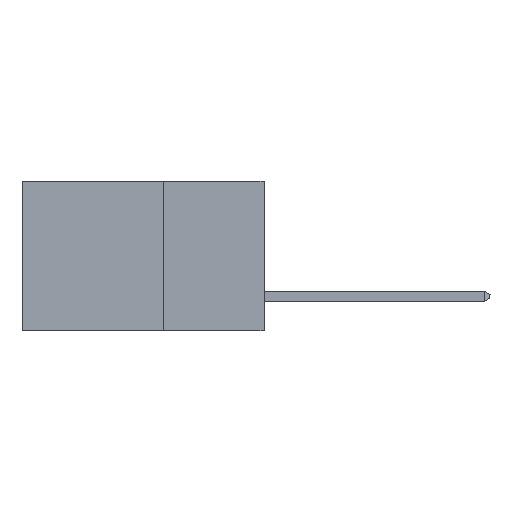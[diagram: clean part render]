
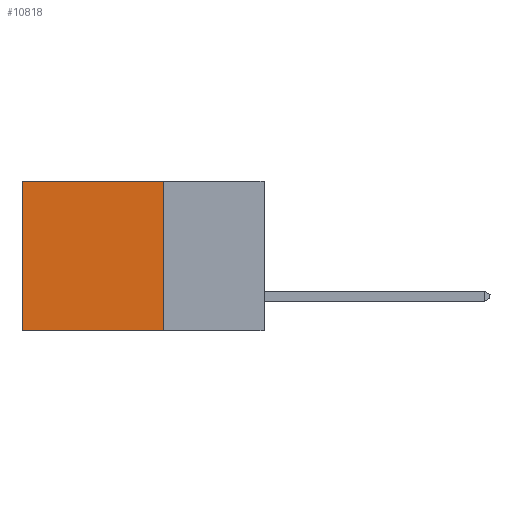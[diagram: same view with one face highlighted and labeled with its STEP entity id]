
A CAD part, left-side view. The second image highlights one B-rep face of the part: STEP entity #10818.
In plain terms, the highlighted planar face has unit normal (-1, 0, 0).
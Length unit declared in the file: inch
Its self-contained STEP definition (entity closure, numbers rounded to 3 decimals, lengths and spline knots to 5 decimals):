
#96 = VERTEX_POINT ( 'NONE', #10178 ) ;
#131 = LINE ( 'NONE', #14228, #1968 ) ;
#228 = AXIS2_PLACEMENT_3D ( 'NONE', #12082, #7778, #13070 ) ;
#303 = VERTEX_POINT ( 'NONE', #3174 ) ;
#800 = EDGE_CURVE ( 'NONE', #96, #4891, #4678, .T. ) ;
#1102 = EDGE_LOOP ( 'NONE', ( #12521, #9415, #10984, #6515 ) ) ;
#1968 = VECTOR ( 'NONE', #13208, 39.37008 ) ;
#2651 = CARTESIAN_POINT ( 'NONE',  ( 0.2615, 0.25, 0. ) ) ;
#3174 = CARTESIAN_POINT ( 'NONE',  ( 0.2615, 0.6, 0. ) ) ;
#3862 = EDGE_CURVE ( 'NONE', #96, #303, #12620, .T. ) ;
#4105 = EDGE_CURVE ( 'NONE', #303, #5831, #13038, .T. ) ;
#4300 = CARTESIAN_POINT ( 'NONE',  ( 0.2615, 0.6, -0.37 ) ) ;
#4678 = LINE ( 'NONE', #9122, #6251 ) ;
#4891 = VERTEX_POINT ( 'NONE', #7332 ) ;
#5831 = VERTEX_POINT ( 'NONE', #4300 ) ;
#6049 = EDGE_CURVE ( 'NONE', #4891, #5831, #131, .T. ) ;
#6251 = VECTOR ( 'NONE', #13386, 39.37008 ) ;
#6460 = FACE_OUTER_BOUND ( 'NONE', #1102, .T. ) ;
#6515 = ORIENTED_EDGE ( 'NONE', *, *, #3862, .T. ) ;
#7098 = DIRECTION ( 'NONE',  ( 0., 1., 0. ) ) ;
#7332 = CARTESIAN_POINT ( 'NONE',  ( 0.2615, 0.25, -0.37 ) ) ;
#7778 = DIRECTION ( 'NONE',  ( 1., 0., 0. ) ) ;
#7781 = VECTOR ( 'NONE', #7098, 39.37008 ) ;
#8678 = CARTESIAN_POINT ( 'NONE',  ( 0.2615, 0.6, -0.37 ) ) ;
#9122 = CARTESIAN_POINT ( 'NONE',  ( 0.2615, 0.25, -0.37 ) ) ;
#9415 = ORIENTED_EDGE ( 'NONE', *, *, #6049, .F. ) ;
#10178 = CARTESIAN_POINT ( 'NONE',  ( 0.2615, 0.25, 0. ) ) ;
#10783 = VECTOR ( 'NONE', #11060, 39.37008 ) ;
#10818 = ADVANCED_FACE ( 'NONE', ( #6460 ), #14167, .F. ) ;
#10984 = ORIENTED_EDGE ( 'NONE', *, *, #800, .F. ) ;
#11060 = DIRECTION ( 'NONE',  ( 0., 0., -1. ) ) ;
#12082 = CARTESIAN_POINT ( 'NONE',  ( 0.2615, 0.25, -0.37 ) ) ;
#12521 = ORIENTED_EDGE ( 'NONE', *, *, #4105, .T. ) ;
#12620 = LINE ( 'NONE', #2651, #7781 ) ;
#13038 = LINE ( 'NONE', #8678, #10783 ) ;
#13070 = DIRECTION ( 'NONE',  ( 0., 0., -1. ) ) ;
#13208 = DIRECTION ( 'NONE',  ( 0., 1., 0. ) ) ;
#13386 = DIRECTION ( 'NONE',  ( 0., 0., -1. ) ) ;
#14167 = PLANE ( 'NONE',  #228 ) ;
#14228 = CARTESIAN_POINT ( 'NONE',  ( 0.2615, 0.25, -0.37 ) ) ;
